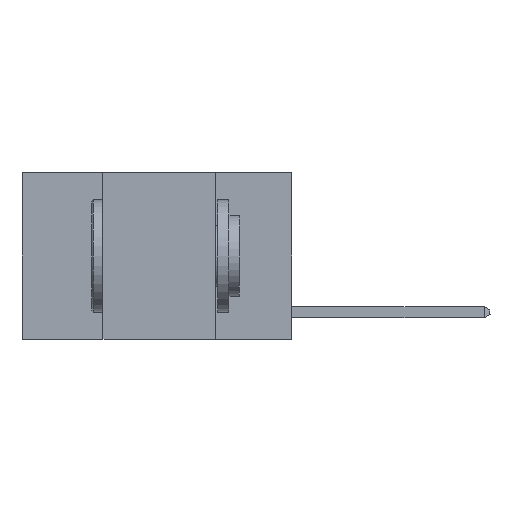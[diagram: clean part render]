
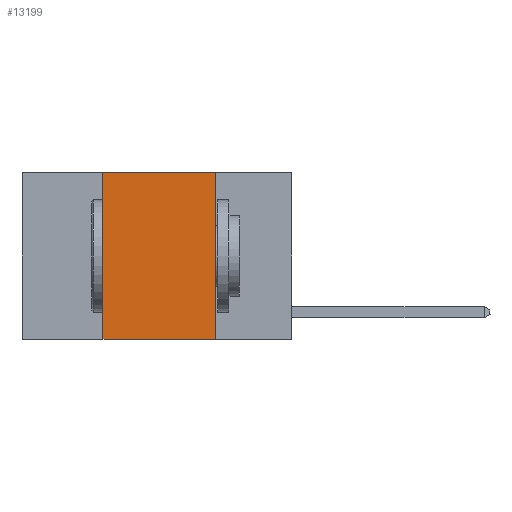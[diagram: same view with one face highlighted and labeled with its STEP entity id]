
A CAD part, left-side view. The second image highlights one B-rep face of the part: STEP entity #13199.
In plain terms, the highlighted planar face has unit normal (-1, 0, 0).
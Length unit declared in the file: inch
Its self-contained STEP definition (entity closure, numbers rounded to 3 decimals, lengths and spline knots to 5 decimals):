
#882 = CARTESIAN_POINT ( 'NONE',  ( 0., 0.17, 0. ) ) ;
#2118 = FACE_OUTER_BOUND ( 'NONE', #23603, .T. ) ;
#2234 = CARTESIAN_POINT ( 'NONE',  ( 0., 0.6, -0.37 ) ) ;
#2272 = DIRECTION ( 'NONE',  ( 0., 0., -1. ) ) ;
#2399 = VERTEX_POINT ( 'NONE', #21779 ) ;
#3325 = VECTOR ( 'NONE', #25992, 39.37008 ) ;
#4091 = EDGE_CURVE ( 'NONE', #24969, #2399, #22095, .T. ) ;
#4432 = PLANE ( 'NONE',  #5359 ) ;
#4794 = LINE ( 'NONE', #882, #13829 ) ;
#5224 = DIRECTION ( 'NONE',  ( 0., 0., -1. ) ) ;
#5359 = AXIS2_PLACEMENT_3D ( 'NONE', #21899, #16878, #2272 ) ;
#6414 = ORIENTED_EDGE ( 'NONE', *, *, #4091, .F. ) ;
#6744 = VERTEX_POINT ( 'NONE', #22045 ) ;
#8259 = DIRECTION ( 'NONE',  ( 0., -1., 0. ) ) ;
#10229 = EDGE_CURVE ( 'NONE', #6744, #20462, #4794, .T. ) ;
#10526 = EDGE_CURVE ( 'NONE', #2399, #6744, #10697, .T. ) ;
#10683 = CARTESIAN_POINT ( 'NONE',  ( 0., 0.42, -0.37 ) ) ;
#10697 = LINE ( 'NONE', #19415, #3325 ) ;
#11315 = VECTOR ( 'NONE', #8259, 39.37008 ) ;
#12713 = VECTOR ( 'NONE', #24785, 39.37008 ) ;
#13199 = ADVANCED_FACE ( 'NONE', ( #2118 ), #4432, .F. ) ;
#13829 = VECTOR ( 'NONE', #5224, 39.37008 ) ;
#15804 = ORIENTED_EDGE ( 'NONE', *, *, #10526, .F. ) ;
#16878 = DIRECTION ( 'NONE',  ( 1., 0., 0. ) ) ;
#19415 = CARTESIAN_POINT ( 'NONE',  ( 0., 0.6, 0. ) ) ;
#20462 = VERTEX_POINT ( 'NONE', #24828 ) ;
#21779 = CARTESIAN_POINT ( 'NONE',  ( 0., 0.42, 0. ) ) ;
#21899 = CARTESIAN_POINT ( 'NONE',  ( 0., 0.6, 0. ) ) ;
#22045 = CARTESIAN_POINT ( 'NONE',  ( 0., 0.17, 0. ) ) ;
#22095 = LINE ( 'NONE', #22519, #12713 ) ;
#22519 = CARTESIAN_POINT ( 'NONE',  ( 0., 0.42, 0. ) ) ;
#23603 = EDGE_LOOP ( 'NONE', ( #27128, #15804, #6414, #28230 ) ) ;
#23712 = LINE ( 'NONE', #2234, #11315 ) ;
#24785 = DIRECTION ( 'NONE',  ( 0., 0., 1. ) ) ;
#24828 = CARTESIAN_POINT ( 'NONE',  ( 0., 0.17, -0.37 ) ) ;
#24969 = VERTEX_POINT ( 'NONE', #10683 ) ;
#25032 = EDGE_CURVE ( 'NONE', #24969, #20462, #23712, .T. ) ;
#25992 = DIRECTION ( 'NONE',  ( 0., -1., 0. ) ) ;
#27128 = ORIENTED_EDGE ( 'NONE', *, *, #10229, .F. ) ;
#28230 = ORIENTED_EDGE ( 'NONE', *, *, #25032, .T. ) ;
